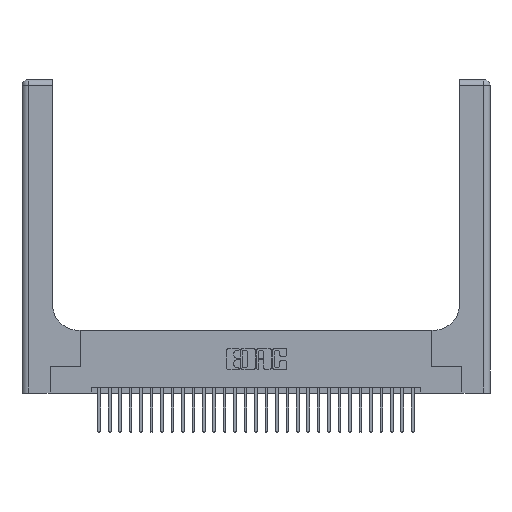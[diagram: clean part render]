
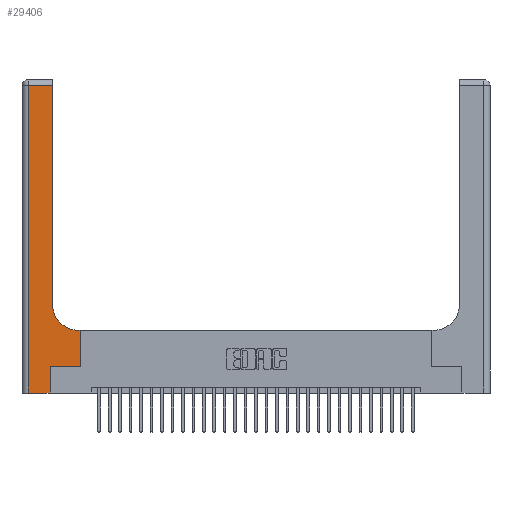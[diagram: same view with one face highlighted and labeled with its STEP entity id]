
A CAD part, top view. The second image highlights one B-rep face of the part: STEP entity #29406.
In plain terms, the highlighted planar face has unit normal (0, 0, 1).
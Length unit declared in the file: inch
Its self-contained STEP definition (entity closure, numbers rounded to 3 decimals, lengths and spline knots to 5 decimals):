
#469 = CARTESIAN_POINT ( 'NONE',  ( 0., 2.94, 0.37 ) ) ;
#788 = LINE ( 'NONE', #26298, #9483 ) ;
#1213 = CARTESIAN_POINT ( 'NONE',  ( 0.2915, 0.6, 0.37 ) ) ;
#2517 = LINE ( 'NONE', #1213, #27283 ) ;
#2556 = CARTESIAN_POINT ( 'NONE',  ( 0.5585, 0.6, 0.37 ) ) ;
#3400 = DIRECTION ( 'NONE',  ( 1., 0., 0. ) ) ;
#3515 = VERTEX_POINT ( 'NONE', #20367 ) ;
#3722 = ORIENTED_EDGE ( 'NONE', *, *, #24680, .T. ) ;
#3792 = VECTOR ( 'NONE', #27132, 39.37008 ) ;
#3971 = AXIS2_PLACEMENT_3D ( 'NONE', #7956, #17571, #5647 ) ;
#4026 = DIRECTION ( 'NONE',  ( 1., 0., 0. ) ) ;
#4238 = VERTEX_POINT ( 'NONE', #27739 ) ;
#4761 = LINE ( 'NONE', #8940, #6635 ) ;
#4889 = LINE ( 'NONE', #469, #3792 ) ;
#5084 = LINE ( 'NONE', #27850, #29816 ) ;
#5647 = DIRECTION ( 'NONE',  ( 1., 0., 0. ) ) ;
#6204 = CARTESIAN_POINT ( 'NONE',  ( 0.2915, 3., 0.37 ) ) ;
#6395 = CARTESIAN_POINT ( 'NONE',  ( 0.269, 0., 0.37 ) ) ;
#6470 = VERTEX_POINT ( 'NONE', #6395 ) ;
#6635 = VECTOR ( 'NONE', #15102, 39.37008 ) ;
#6881 = ORIENTED_EDGE ( 'NONE', *, *, #8908, .T. ) ;
#7956 = CARTESIAN_POINT ( 'NONE',  ( 0.5415, 0.85, 0.37 ) ) ;
#8283 = DIRECTION ( 'NONE',  ( -1., 0., 0. ) ) ;
#8908 = EDGE_CURVE ( 'NONE', #3515, #23692, #19439, .T. ) ;
#8940 = CARTESIAN_POINT ( 'NONE',  ( 0.06, 3., 0.37 ) ) ;
#8959 = VECTOR ( 'NONE', #18128, 39.37008 ) ;
#9056 = CARTESIAN_POINT ( 'NONE',  ( 0.06, 0., 0.37 ) ) ;
#9111 = EDGE_LOOP ( 'NONE', ( #6881, #22292, #9170, #28083, #15514, #26920, #3722, #13906, #10630 ) ) ;
#9170 = ORIENTED_EDGE ( 'NONE', *, *, #19172, .T. ) ;
#9280 = EDGE_CURVE ( 'NONE', #14586, #23097, #2517, .T. ) ;
#9332 = DIRECTION ( 'NONE',  ( 0., 1., 0. ) ) ;
#9483 = VECTOR ( 'NONE', #3400, 39.37008 ) ;
#10630 = ORIENTED_EDGE ( 'NONE', *, *, #26330, .T. ) ;
#10832 = CARTESIAN_POINT ( 'NONE',  ( 0.5415, 0.6, 0.37 ) ) ;
#11683 = DIRECTION ( 'NONE',  ( 0., 0., -1. ) ) ;
#13906 = ORIENTED_EDGE ( 'NONE', *, *, #9280, .T. ) ;
#14024 = PLANE ( 'NONE',  #27692 ) ;
#14586 = VERTEX_POINT ( 'NONE', #2556 ) ;
#15102 = DIRECTION ( 'NONE',  ( 0., -1., 0. ) ) ;
#15514 = ORIENTED_EDGE ( 'NONE', *, *, #27779, .T. ) ;
#15816 = EDGE_CURVE ( 'NONE', #21252, #6470, #788, .T. ) ;
#15957 = CARTESIAN_POINT ( 'NONE',  ( 0.269, 0.25, 0.37 ) ) ;
#17571 = DIRECTION ( 'NONE',  ( 0., 0., -1. ) ) ;
#18128 = DIRECTION ( 'NONE',  ( 0., 1., 0. ) ) ;
#18183 = CARTESIAN_POINT ( 'NONE',  ( 0.5585, 0.25, 0.37 ) ) ;
#18717 = CARTESIAN_POINT ( 'NONE',  ( 0., 3., 0.37 ) ) ;
#19172 = EDGE_CURVE ( 'NONE', #4238, #21252, #4761, .T. ) ;
#19439 = LINE ( 'NONE', #6204, #8959 ) ;
#20367 = CARTESIAN_POINT ( 'NONE',  ( 0.2915, 0.85, 0.37 ) ) ;
#20391 = VECTOR ( 'NONE', #9332, 39.37008 ) ;
#21252 = VERTEX_POINT ( 'NONE', #9056 ) ;
#21511 = FACE_OUTER_BOUND ( 'NONE', #9111, .T. ) ;
#21548 = LINE ( 'NONE', #22989, #21878 ) ;
#21646 = CARTESIAN_POINT ( 'NONE',  ( 0.2915, 2.94, 0.37 ) ) ;
#21878 = VECTOR ( 'NONE', #4026, 39.37008 ) ;
#22292 = ORIENTED_EDGE ( 'NONE', *, *, #26896, .T. ) ;
#22989 = CARTESIAN_POINT ( 'NONE',  ( 0.269, 0.25, 0.37 ) ) ;
#23097 = VERTEX_POINT ( 'NONE', #10832 ) ;
#23615 = CARTESIAN_POINT ( 'NONE',  ( 0.5585, 0.25, 0.37 ) ) ;
#23692 = VERTEX_POINT ( 'NONE', #21646 ) ;
#24054 = VERTEX_POINT ( 'NONE', #15957 ) ;
#24104 = EDGE_CURVE ( 'NONE', #24054, #27611, #21548, .T. ) ;
#24680 = EDGE_CURVE ( 'NONE', #27611, #14586, #26772, .T. ) ;
#25985 = DIRECTION ( 'NONE',  ( -1., 0., 0. ) ) ;
#26298 = CARTESIAN_POINT ( 'NONE',  ( 0., 0., 0.37 ) ) ;
#26330 = EDGE_CURVE ( 'NONE', #23097, #3515, #28589, .T. ) ;
#26772 = LINE ( 'NONE', #23615, #20391 ) ;
#26896 = EDGE_CURVE ( 'NONE', #23692, #4238, #4889, .T. ) ;
#26920 = ORIENTED_EDGE ( 'NONE', *, *, #24104, .T. ) ;
#27132 = DIRECTION ( 'NONE',  ( -1., 0., 0. ) ) ;
#27283 = VECTOR ( 'NONE', #8283, 39.37008 ) ;
#27611 = VERTEX_POINT ( 'NONE', #18183 ) ;
#27692 = AXIS2_PLACEMENT_3D ( 'NONE', #18717, #11683, #25985 ) ;
#27739 = CARTESIAN_POINT ( 'NONE',  ( 0.06, 2.94, 0.37 ) ) ;
#27779 = EDGE_CURVE ( 'NONE', #6470, #24054, #5084, .T. ) ;
#27850 = CARTESIAN_POINT ( 'NONE',  ( 0.269, 0., 0.37 ) ) ;
#28083 = ORIENTED_EDGE ( 'NONE', *, *, #15816, .T. ) ;
#28366 = DIRECTION ( 'NONE',  ( 0., 1., 0. ) ) ;
#28589 = CIRCLE ( 'NONE', #3971, 0.25 ) ;
#29406 = ADVANCED_FACE ( 'NONE', ( #21511 ), #14024, .F. ) ;
#29816 = VECTOR ( 'NONE', #28366, 39.37008 ) ;
